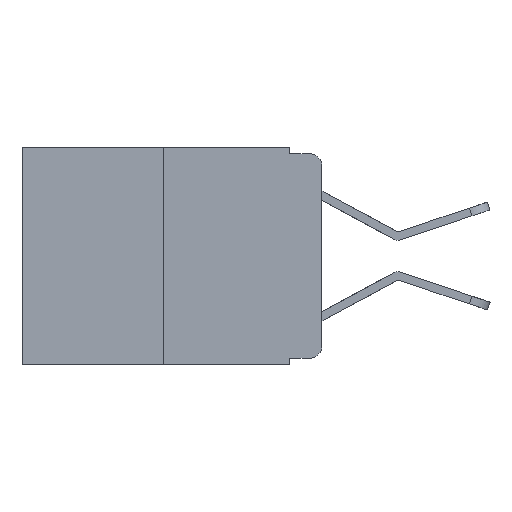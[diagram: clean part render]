
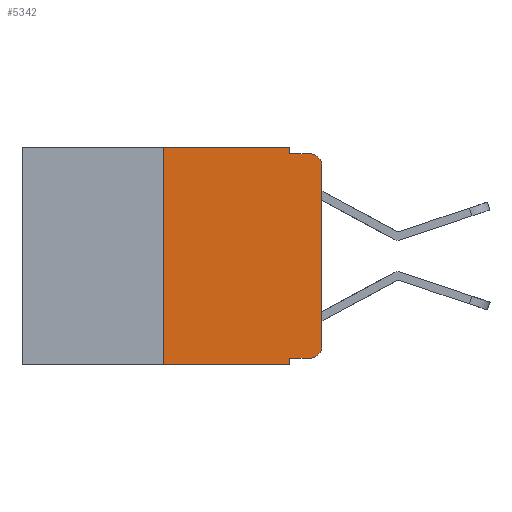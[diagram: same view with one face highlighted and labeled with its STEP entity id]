
A CAD part, left-side view. The second image highlights one B-rep face of the part: STEP entity #5342.
In plain terms, the highlighted planar face has unit normal (-1, 0, 0).
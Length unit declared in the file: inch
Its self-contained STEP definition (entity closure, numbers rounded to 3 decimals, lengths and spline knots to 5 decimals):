
#93 = CARTESIAN_POINT ( 'NONE',  ( 0., 0.25, 0. ) ) ;
#186 = VERTEX_POINT ( 'NONE', #14373 ) ;
#232 = CARTESIAN_POINT ( 'NONE',  ( 0., 0.02, -0.333 ) ) ;
#602 = CARTESIAN_POINT ( 'NONE',  ( 0., 0.051, 0. ) ) ;
#734 = CARTESIAN_POINT ( 'NONE',  ( 0., 0.473, 0. ) ) ;
#953 = LINE ( 'NONE', #4504, #9612 ) ;
#962 = ORIENTED_EDGE ( 'NONE', *, *, #8232, .T. ) ;
#1026 = EDGE_CURVE ( 'NONE', #8612, #12203, #953, .T. ) ;
#1116 = VERTEX_POINT ( 'NONE', #1235 ) ;
#1207 = ORIENTED_EDGE ( 'NONE', *, *, #4695, .F. ) ;
#1235 = CARTESIAN_POINT ( 'NONE',  ( 0., 0.051, 0. ) ) ;
#1821 = LINE ( 'NONE', #2897, #4661 ) ;
#2415 = CARTESIAN_POINT ( 'NONE',  ( 0., 0.02, -0.03 ) ) ;
#2897 = CARTESIAN_POINT ( 'NONE',  ( 0., 0.473, 0. ) ) ;
#2935 = CARTESIAN_POINT ( 'NONE',  ( 0., 0., -0.03 ) ) ;
#2949 = ORIENTED_EDGE ( 'NONE', *, *, #9184, .T. ) ;
#3153 = CARTESIAN_POINT ( 'NONE',  ( 0., 0.473, -0.343 ) ) ;
#3516 = VERTEX_POINT ( 'NONE', #8590 ) ;
#3614 = ORIENTED_EDGE ( 'NONE', *, *, #6531, .F. ) ;
#4245 = VERTEX_POINT ( 'NONE', #13629 ) ;
#4286 = FACE_OUTER_BOUND ( 'NONE', #6746, .T. ) ;
#4288 = ORIENTED_EDGE ( 'NONE', *, *, #13747, .F. ) ;
#4504 = CARTESIAN_POINT ( 'NONE',  ( 0., 0., 0. ) ) ;
#4651 = VECTOR ( 'NONE', #8840, 39.37008 ) ;
#4661 = VECTOR ( 'NONE', #12183, 39.37008 ) ;
#4695 = EDGE_CURVE ( 'NONE', #186, #6997, #11862, .T. ) ;
#5034 = DIRECTION ( 'NONE',  ( 0., -1., 0. ) ) ;
#5342 = ADVANCED_FACE ( 'NONE', ( #4286 ), #7942, .F. ) ;
#5381 = EDGE_CURVE ( 'NONE', #186, #11495, #5494, .T. ) ;
#5494 = LINE ( 'NONE', #3153, #12113 ) ;
#5768 = ORIENTED_EDGE ( 'NONE', *, *, #10044, .F. ) ;
#5828 = VECTOR ( 'NONE', #5034, 39.37008 ) ;
#6168 = LINE ( 'NONE', #10802, #5828 ) ;
#6531 = EDGE_CURVE ( 'NONE', #4245, #11495, #9463, .T. ) ;
#6555 = AXIS2_PLACEMENT_3D ( 'NONE', #2415, #7024, #14124 ) ;
#6746 = EDGE_LOOP ( 'NONE', ( #9560, #14194, #4288, #5768, #9193, #1207, #9606, #3614, #2949, #962 ) ) ;
#6997 = VERTEX_POINT ( 'NONE', #12808 ) ;
#7024 = DIRECTION ( 'NONE',  ( -1., 0., 0. ) ) ;
#7701 = CARTESIAN_POINT ( 'NONE',  ( 0., 0.051, -0.333 ) ) ;
#7827 = VERTEX_POINT ( 'NONE', #9836 ) ;
#7864 = DIRECTION ( 'NONE',  ( 0., -1., 0. ) ) ;
#7942 = PLANE ( 'NONE',  #9724 ) ;
#8232 = EDGE_CURVE ( 'NONE', #13223, #8612, #10445, .T. ) ;
#8590 = CARTESIAN_POINT ( 'NONE',  ( 0., 0.051, -0.01 ) ) ;
#8612 = VERTEX_POINT ( 'NONE', #10665 ) ;
#8840 = DIRECTION ( 'NONE',  ( 0., -1., 0. ) ) ;
#8859 = LINE ( 'NONE', #602, #14078 ) ;
#8929 = DIRECTION ( 'NONE',  ( 0., 0., -1. ) ) ;
#9184 = EDGE_CURVE ( 'NONE', #4245, #13223, #14318, .T. ) ;
#9193 = ORIENTED_EDGE ( 'NONE', *, *, #13012, .F. ) ;
#9326 = DIRECTION ( 'NONE',  ( 0., 0., 1. ) ) ;
#9463 = LINE ( 'NONE', #13053, #14589 ) ;
#9483 = DIRECTION ( 'NONE',  ( 0., 0., -1. ) ) ;
#9560 = ORIENTED_EDGE ( 'NONE', *, *, #1026, .T. ) ;
#9606 = ORIENTED_EDGE ( 'NONE', *, *, #5381, .T. ) ;
#9612 = VECTOR ( 'NONE', #11233, 39.37008 ) ;
#9698 = DIRECTION ( 'NONE',  ( -1., 0., 0. ) ) ;
#9724 = AXIS2_PLACEMENT_3D ( 'NONE', #734, #10047, #13502 ) ;
#9836 = CARTESIAN_POINT ( 'NONE',  ( 0., 0.02, -0.01 ) ) ;
#10044 = EDGE_CURVE ( 'NONE', #1116, #3516, #8859, .T. ) ;
#10047 = DIRECTION ( 'NONE',  ( 1., 0., 0. ) ) ;
#10234 = CARTESIAN_POINT ( 'NONE',  ( 0., 0.051, -0.343 ) ) ;
#10445 = CIRCLE ( 'NONE', #13789, 0.02 ) ;
#10665 = CARTESIAN_POINT ( 'NONE',  ( 0., 0., -0.313 ) ) ;
#10802 = CARTESIAN_POINT ( 'NONE',  ( 0., 0.051, -0.01 ) ) ;
#11053 = VECTOR ( 'NONE', #9326, 39.37008 ) ;
#11233 = DIRECTION ( 'NONE',  ( 0., 0., 1. ) ) ;
#11495 = VERTEX_POINT ( 'NONE', #10234 ) ;
#11722 = EDGE_CURVE ( 'NONE', #12203, #7827, #14255, .T. ) ;
#11782 = DIRECTION ( 'NONE',  ( 0., 0., -1. ) ) ;
#11862 = LINE ( 'NONE', #93, #11053 ) ;
#12113 = VECTOR ( 'NONE', #7864, 39.37008 ) ;
#12183 = DIRECTION ( 'NONE',  ( 0., -1., 0. ) ) ;
#12203 = VERTEX_POINT ( 'NONE', #2935 ) ;
#12808 = CARTESIAN_POINT ( 'NONE',  ( 0., 0.25, 0. ) ) ;
#13012 = EDGE_CURVE ( 'NONE', #6997, #1116, #1821, .T. ) ;
#13053 = CARTESIAN_POINT ( 'NONE',  ( 0., 0.051, 0. ) ) ;
#13223 = VERTEX_POINT ( 'NONE', #232 ) ;
#13502 = DIRECTION ( 'NONE',  ( 0., 0., -1. ) ) ;
#13629 = CARTESIAN_POINT ( 'NONE',  ( 0., 0.051, -0.333 ) ) ;
#13747 = EDGE_CURVE ( 'NONE', #3516, #7827, #6168, .T. ) ;
#13789 = AXIS2_PLACEMENT_3D ( 'NONE', #14140, #9698, #9483 ) ;
#14078 = VECTOR ( 'NONE', #8929, 39.37008 ) ;
#14124 = DIRECTION ( 'NONE',  ( 0., 0., -1. ) ) ;
#14140 = CARTESIAN_POINT ( 'NONE',  ( 0., 0.02, -0.313 ) ) ;
#14194 = ORIENTED_EDGE ( 'NONE', *, *, #11722, .T. ) ;
#14255 = CIRCLE ( 'NONE', #6555, 0.02 ) ;
#14318 = LINE ( 'NONE', #7701, #4651 ) ;
#14373 = CARTESIAN_POINT ( 'NONE',  ( 0., 0.25, -0.343 ) ) ;
#14589 = VECTOR ( 'NONE', #11782, 39.37008 ) ;
